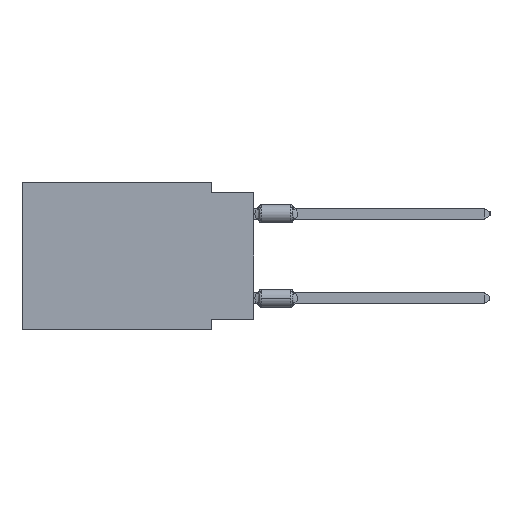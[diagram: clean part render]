
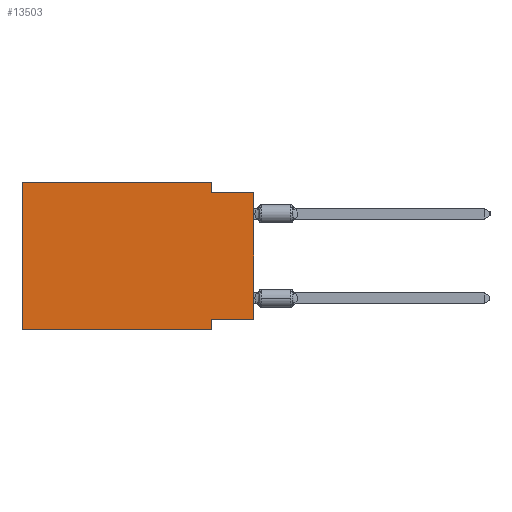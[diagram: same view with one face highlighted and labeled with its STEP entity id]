
A CAD part, left-side view. The second image highlights one B-rep face of the part: STEP entity #13503.
In plain terms, the highlighted planar face has unit normal (-1, 0, 0).
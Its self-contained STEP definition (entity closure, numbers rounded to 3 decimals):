
#608 = ORIENTED_EDGE ( 'NONE', *, *, #52741, .F. ) ;
#1316 = LINE ( 'NONE', #54834, #39250 ) ;
#1426 = ORIENTED_EDGE ( 'NONE', *, *, #25987, .T. ) ;
#3505 = CARTESIAN_POINT ( 'NONE',  ( 0., 0., -8.255 ) ) ;
#4619 = ORIENTED_EDGE ( 'NONE', *, *, #50158, .F. ) ;
#4734 = DIRECTION ( 'NONE',  ( 0., 0., -1. ) ) ;
#5024 = CARTESIAN_POINT ( 'NONE',  ( 0., 2.54, -8.255 ) ) ;
#5331 = CARTESIAN_POINT ( 'NONE',  ( 0., 0., -0.635 ) ) ;
#6672 = DIRECTION ( 'NONE',  ( 0., -1., 0. ) ) ;
#7535 = CARTESIAN_POINT ( 'NONE',  ( 0., 2.54, -8.89 ) ) ;
#9842 = DIRECTION ( 'NONE',  ( 0., -1., 0. ) ) ;
#11652 = VERTEX_POINT ( 'NONE', #5024 ) ;
#11946 = DIRECTION ( 'NONE',  ( 0., 0., -1. ) ) ;
#12713 = CARTESIAN_POINT ( 'NONE',  ( 0., 13.97, -8.89 ) ) ;
#13482 = CARTESIAN_POINT ( 'NONE',  ( 0., 0., 0. ) ) ;
#13503 = ADVANCED_FACE ( 'NONE', ( #36328 ), #31939, .F. ) ;
#14400 = LINE ( 'NONE', #5331, #25046 ) ;
#14429 = EDGE_CURVE ( 'NONE', #16866, #42856, #18908, .T. ) ;
#14750 = DIRECTION ( 'NONE',  ( 0., 0., -1. ) ) ;
#16866 = VERTEX_POINT ( 'NONE', #52819 ) ;
#17033 = LINE ( 'NONE', #48908, #31071 ) ;
#18156 = DIRECTION ( 'NONE',  ( 0., 0., 1. ) ) ;
#18908 = LINE ( 'NONE', #26803, #54546 ) ;
#22618 = VERTEX_POINT ( 'NONE', #3505 ) ;
#22850 = CARTESIAN_POINT ( 'NONE',  ( 0., 13.97, 0. ) ) ;
#23056 = EDGE_CURVE ( 'NONE', #11652, #30540, #34455, .T. ) ;
#23538 = VECTOR ( 'NONE', #6672, 1000. ) ;
#24510 = ORIENTED_EDGE ( 'NONE', *, *, #28177, .F. ) ;
#25046 = VECTOR ( 'NONE', #49812, 1000. ) ;
#25577 = DIRECTION ( 'NONE',  ( 0., 0., 1. ) ) ;
#25987 = EDGE_CURVE ( 'NONE', #36860, #30540, #41768, .T. ) ;
#26332 = VECTOR ( 'NONE', #36418, 1000. ) ;
#26466 = EDGE_LOOP ( 'NONE', ( #36099, #608, #30710, #38317, #24510, #1426, #32392, #4619 ) ) ;
#26803 = CARTESIAN_POINT ( 'NONE',  ( 0., 13.97, 0. ) ) ;
#28177 = EDGE_CURVE ( 'NONE', #36860, #16866, #17033, .T. ) ;
#28327 = CARTESIAN_POINT ( 'NONE',  ( 0., 13.97, -8.89 ) ) ;
#29208 = CARTESIAN_POINT ( 'NONE',  ( 0., 2.54, -8.89 ) ) ;
#30176 = AXIS2_PLACEMENT_3D ( 'NONE', #22850, #40430, #4734 ) ;
#30186 = CARTESIAN_POINT ( 'NONE',  ( 0., 2.54, 0. ) ) ;
#30540 = VERTEX_POINT ( 'NONE', #7535 ) ;
#30710 = ORIENTED_EDGE ( 'NONE', *, *, #53596, .F. ) ;
#31071 = VECTOR ( 'NONE', #18156, 1000. ) ;
#31741 = LINE ( 'NONE', #49290, #26332 ) ;
#31939 = PLANE ( 'NONE',  #30176 ) ;
#32392 = ORIENTED_EDGE ( 'NONE', *, *, #23056, .F. ) ;
#34233 = VERTEX_POINT ( 'NONE', #45247 ) ;
#34455 = LINE ( 'NONE', #29208, #45196 ) ;
#36061 = CARTESIAN_POINT ( 'NONE',  ( 0., 2.54, -0.635 ) ) ;
#36099 = ORIENTED_EDGE ( 'NONE', *, *, #38339, .T. ) ;
#36328 = FACE_OUTER_BOUND ( 'NONE', #26466, .T. ) ;
#36418 = DIRECTION ( 'NONE',  ( 0., 1., 0. ) ) ;
#36860 = VERTEX_POINT ( 'NONE', #12713 ) ;
#38317 = ORIENTED_EDGE ( 'NONE', *, *, #14429, .F. ) ;
#38339 = EDGE_CURVE ( 'NONE', #22618, #34233, #56588, .T. ) ;
#39250 = VECTOR ( 'NONE', #14750, 1000. ) ;
#40430 = DIRECTION ( 'NONE',  ( 1., 0., 0. ) ) ;
#41171 = VERTEX_POINT ( 'NONE', #36061 ) ;
#41768 = LINE ( 'NONE', #28327, #23538 ) ;
#42856 = VERTEX_POINT ( 'NONE', #30186 ) ;
#45196 = VECTOR ( 'NONE', #11946, 1000. ) ;
#45247 = CARTESIAN_POINT ( 'NONE',  ( 0., 0., -0.635 ) ) ;
#46540 = VECTOR ( 'NONE', #25577, 1000. ) ;
#48908 = CARTESIAN_POINT ( 'NONE',  ( 0., 13.97, 0. ) ) ;
#49290 = CARTESIAN_POINT ( 'NONE',  ( 0., 0., -8.255 ) ) ;
#49812 = DIRECTION ( 'NONE',  ( 0., -1., 0. ) ) ;
#50158 = EDGE_CURVE ( 'NONE', #22618, #11652, #31741, .T. ) ;
#52741 = EDGE_CURVE ( 'NONE', #41171, #34233, #14400, .T. ) ;
#52819 = CARTESIAN_POINT ( 'NONE',  ( 0., 13.97, 0. ) ) ;
#53596 = EDGE_CURVE ( 'NONE', #42856, #41171, #1316, .T. ) ;
#54546 = VECTOR ( 'NONE', #9842, 1000. ) ;
#54834 = CARTESIAN_POINT ( 'NONE',  ( 0., 2.54, 0. ) ) ;
#56588 = LINE ( 'NONE', #13482, #46540 ) ;
